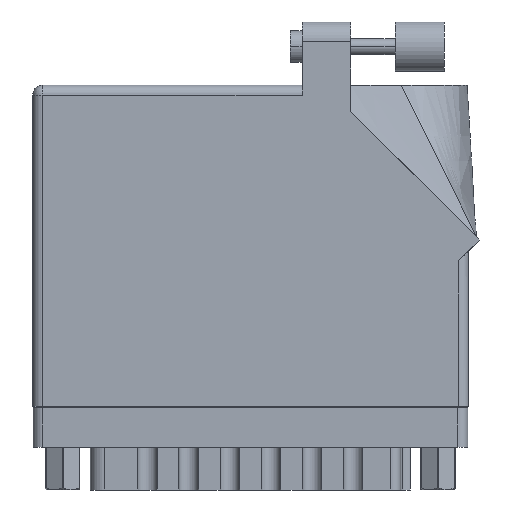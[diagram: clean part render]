
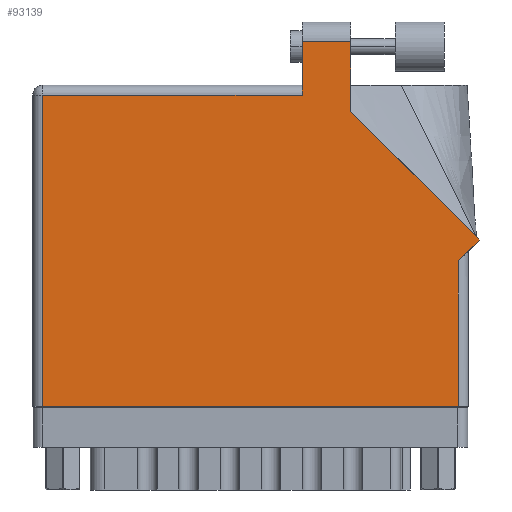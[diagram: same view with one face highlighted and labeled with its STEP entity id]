
A CAD part, front view. The second image highlights one B-rep face of the part: STEP entity #93139.
In plain terms, the highlighted face is planar.
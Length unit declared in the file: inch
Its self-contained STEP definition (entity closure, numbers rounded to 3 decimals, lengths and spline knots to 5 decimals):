
#521 = CARTESIAN_POINT ( 'NONE',  ( 2.755, 0.98, 0. ) ) ;
#4764 = VECTOR ( 'NONE', #39918, 39.37008 ) ;
#5779 = ORIENTED_EDGE ( 'NONE', *, *, #47308, .T. ) ;
#8455 = DIRECTION ( 'NONE',  ( -1., 0., 0. ) ) ;
#8837 = EDGE_CURVE ( 'NONE', #78240, #76449, #43201, .T. ) ;
#19618 = CARTESIAN_POINT ( 'NONE',  ( 2.693, 0.918, 0. ) ) ;
#20306 = EDGE_CURVE ( 'NONE', #57626, #47920, #47929, .T. ) ;
#21364 = ORIENTED_EDGE ( 'NONE', *, *, #98260, .T. ) ;
#22704 = DIRECTION ( 'NONE',  ( 0.707, 0.707, 0. ) ) ;
#25379 = CARTESIAN_POINT ( 'NONE',  ( 2.012, 2.305, 0. ) ) ;
#26432 = ORIENTED_EDGE ( 'NONE', *, *, #8837, .T. ) ;
#26812 = LINE ( 'NONE', #74612, #56851 ) ;
#28634 = DIRECTION ( 'NONE',  ( -0.707, 0.707, 0. ) ) ;
#29828 = CARTESIAN_POINT ( 'NONE',  ( 2.82571, 1.05071, 0. ) ) ;
#30419 = ORIENTED_EDGE ( 'NONE', *, *, #20306, .T. ) ;
#31969 = DIRECTION ( 'NONE',  ( 0., 1., 0. ) ) ;
#33525 = VERTEX_POINT ( 'NONE', #57865 ) ;
#34079 = EDGE_CURVE ( 'NONE', #76449, #44614, #40152, .T. ) ;
#35683 = FACE_OUTER_BOUND ( 'NONE', #59750, .T. ) ;
#35954 = PLANE ( 'NONE',  #48047 ) ;
#36307 = CARTESIAN_POINT ( 'NONE',  ( 2.693, 0., 0. ) ) ;
#37465 = CARTESIAN_POINT ( 'NONE',  ( 0.062, 0., 0. ) ) ;
#38924 = CARTESIAN_POINT ( 'NONE',  ( 0., 1.968, 0. ) ) ;
#39918 = DIRECTION ( 'NONE',  ( -1., 0., 0. ) ) ;
#40152 = LINE ( 'NONE', #521, #46105 ) ;
#41162 = DIRECTION ( 'NONE',  ( 0., 1., 0. ) ) ;
#41821 = VERTEX_POINT ( 'NONE', #61888 ) ;
#43201 = LINE ( 'NONE', #48208, #76833 ) ;
#44614 = VERTEX_POINT ( 'NONE', #29828 ) ;
#46105 = VECTOR ( 'NONE', #22704, 39.37008 ) ;
#47308 = EDGE_CURVE ( 'NONE', #50730, #33525, #84209, .T. ) ;
#47412 = CARTESIAN_POINT ( 'NONE',  ( 0., 0., 0. ) ) ;
#47430 = CARTESIAN_POINT ( 'NONE',  ( 1.705, 2.03, 0. ) ) ;
#47920 = VERTEX_POINT ( 'NONE', #25379 ) ;
#47929 = LINE ( 'NONE', #54797, #52736 ) ;
#48047 = AXIS2_PLACEMENT_3D ( 'NONE', #72879, #89345, #96755 ) ;
#48208 = CARTESIAN_POINT ( 'NONE',  ( 2.693, 0.98, 0. ) ) ;
#48712 = LINE ( 'NONE', #47430, #55943 ) ;
#50730 = VERTEX_POINT ( 'NONE', #85852 ) ;
#52736 = VECTOR ( 'NONE', #31969, 39.37008 ) ;
#54797 = CARTESIAN_POINT ( 'NONE',  ( 2.012, 1.86442, 0. ) ) ;
#55896 = ORIENTED_EDGE ( 'NONE', *, *, #84111, .T. ) ;
#55943 = VECTOR ( 'NONE', #69946, 39.37008 ) ;
#56851 = VECTOR ( 'NONE', #28634, 39.37008 ) ;
#57626 = VERTEX_POINT ( 'NONE', #84895 ) ;
#57865 = CARTESIAN_POINT ( 'NONE',  ( 0.062, 1.968, 0. ) ) ;
#57949 = LINE ( 'NONE', #47412, #84389 ) ;
#59750 = EDGE_LOOP ( 'NONE', ( #30419, #87354, #62514, #5779, #21364, #61176, #26432, #76447, #55896 ) ) ;
#61176 = ORIENTED_EDGE ( 'NONE', *, *, #73198, .T. ) ;
#61318 = VECTOR ( 'NONE', #8455, 39.37008 ) ;
#61888 = CARTESIAN_POINT ( 'NONE',  ( 1.705, 2.305, 0. ) ) ;
#62514 = ORIENTED_EDGE ( 'NONE', *, *, #77835, .T. ) ;
#63520 = DIRECTION ( 'NONE',  ( 1., 0., 0. ) ) ;
#65927 = LINE ( 'NONE', #37465, #79114 ) ;
#69946 = DIRECTION ( 'NONE',  ( 0., -1., 0. ) ) ;
#70172 = CARTESIAN_POINT ( 'NONE',  ( 1.705, 2.305, 0. ) ) ;
#72879 = CARTESIAN_POINT ( 'NONE',  ( 0., 2.03, 0. ) ) ;
#73198 = EDGE_CURVE ( 'NONE', #91000, #78240, #57949, .T. ) ;
#74612 = CARTESIAN_POINT ( 'NONE',  ( 2.82571, 1.05071, 0. ) ) ;
#76447 = ORIENTED_EDGE ( 'NONE', *, *, #34079, .T. ) ;
#76449 = VERTEX_POINT ( 'NONE', #19618 ) ;
#76833 = VECTOR ( 'NONE', #41162, 39.37008 ) ;
#77835 = EDGE_CURVE ( 'NONE', #41821, #50730, #48712, .T. ) ;
#78240 = VERTEX_POINT ( 'NONE', #36307 ) ;
#79114 = VECTOR ( 'NONE', #82837, 39.37008 ) ;
#79389 = CARTESIAN_POINT ( 'NONE',  ( 0.062, 0., 0. ) ) ;
#79947 = EDGE_CURVE ( 'NONE', #47920, #41821, #84035, .T. ) ;
#82837 = DIRECTION ( 'NONE',  ( 0., -1., 0. ) ) ;
#84035 = LINE ( 'NONE', #70172, #4764 ) ;
#84111 = EDGE_CURVE ( 'NONE', #44614, #57626, #26812, .T. ) ;
#84209 = LINE ( 'NONE', #38924, #61318 ) ;
#84389 = VECTOR ( 'NONE', #63520, 39.37008 ) ;
#84895 = CARTESIAN_POINT ( 'NONE',  ( 2.012, 1.86442, 0. ) ) ;
#85852 = CARTESIAN_POINT ( 'NONE',  ( 1.705, 1.968, 0. ) ) ;
#87354 = ORIENTED_EDGE ( 'NONE', *, *, #79947, .T. ) ;
#89345 = DIRECTION ( 'NONE',  ( 0., 0., -1. ) ) ;
#91000 = VERTEX_POINT ( 'NONE', #79389 ) ;
#93139 = ADVANCED_FACE ( 'NONE', ( #35683 ), #35954, .F. ) ;
#96755 = DIRECTION ( 'NONE',  ( -1., 0., 0. ) ) ;
#98260 = EDGE_CURVE ( 'NONE', #33525, #91000, #65927, .T. ) ;
